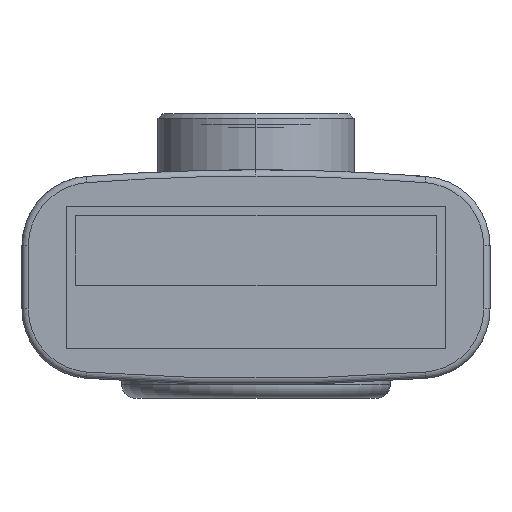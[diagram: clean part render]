
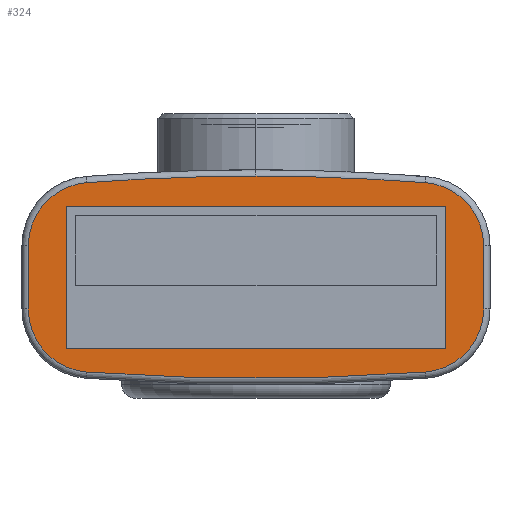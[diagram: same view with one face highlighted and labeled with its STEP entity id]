
A CAD part, front view. The second image highlights one B-rep face of the part: STEP entity #324.
In plain terms, the highlighted planar face has unit normal (0, -1, 0).
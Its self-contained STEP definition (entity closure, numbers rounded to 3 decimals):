
#100 = LINE ( 'NONE', #1617, #2798 ) ;
#133 = CARTESIAN_POINT ( 'NONE',  ( 54.8, -186.8, -10.175 ) ) ;
#142 = CARTESIAN_POINT ( 'NONE',  ( 52.8, -186.8, -12.175 ) ) ;
#231 = AXIS2_PLACEMENT_3D ( 'NONE', #3748, #353, #1868 ) ;
#239 = DIRECTION ( 'NONE',  ( 0., 1., 0. ) ) ;
#260 = CIRCLE ( 'NONE', #338, 69.8 ) ;
#324 = ADVANCED_FACE ( 'NONE', ( #4013, #614 ), #2124, .F. ) ;
#338 = AXIS2_PLACEMENT_3D ( 'NONE', #1811, #3325, #4828 ) ;
#353 = DIRECTION ( 'NONE',  ( 0., 1., 0. ) ) ;
#392 = DIRECTION ( 'NONE',  ( -0.075, 0., -0.997 ) ) ;
#433 = EDGE_CURVE ( 'NONE', #1878, #1006, #3667, .T. ) ;
#448 = CARTESIAN_POINT ( 'NONE',  ( 54., -186.8, -13.425 ) ) ;
#493 = EDGE_CURVE ( 'NONE', #609, #1517, #1768, .T. ) ;
#539 = EDGE_CURVE ( 'NONE', #4317, #609, #260, .T. ) ;
#552 = VERTEX_POINT ( 'NONE', #4093 ) ;
#590 = CARTESIAN_POINT ( 'NONE',  ( 65.2, -186.8, -12.175 ) ) ;
#595 = VERTEX_POINT ( 'NONE', #2628 ) ;
#609 = VERTEX_POINT ( 'NONE', #3400 ) ;
#614 = FACE_BOUND ( 'NONE', #2834, .T. ) ;
#627 = CARTESIAN_POINT ( 'NONE',  ( 52.8, -186.8, -10.176 ) ) ;
#640 = CIRCLE ( 'NONE', #231, 69.8 ) ;
#694 = ORIENTED_EDGE ( 'NONE', *, *, #539, .F. ) ;
#700 = CARTESIAN_POINT ( 'NONE',  ( 65.353, -186.8, -8.181 ) ) ;
#705 = VERTEX_POINT ( 'NONE', #2711 ) ;
#777 = LINE ( 'NONE', #2286, #2953 ) ;
#838 = ORIENTED_EDGE ( 'NONE', *, *, #433, .F. ) ;
#866 = AXIS2_PLACEMENT_3D ( 'NONE', #3635, #239, #1753 ) ;
#899 = DIRECTION ( 'NONE',  ( 0., 0., 1. ) ) ;
#978 = ORIENTED_EDGE ( 'NONE', *, *, #2802, .F. ) ;
#1006 = VERTEX_POINT ( 'NONE', #2347 ) ;
#1067 = AXIS2_PLACEMENT_3D ( 'NONE', #4663, #1274, #2794 ) ;
#1149 = CIRCLE ( 'NONE', #1067, 2. ) ;
#1180 = VERTEX_POINT ( 'NONE', #700 ) ;
#1221 = CARTESIAN_POINT ( 'NONE',  ( 67.2, -186.8, -10.175 ) ) ;
#1274 = DIRECTION ( 'NONE',  ( 0., 1., 0. ) ) ;
#1292 = VECTOR ( 'NONE', #899, 1000. ) ;
#1330 = VERTEX_POINT ( 'NONE', #1221 ) ;
#1357 = EDGE_CURVE ( 'NONE', #4426, #552, #100, .T. ) ;
#1362 = CIRCLE ( 'NONE', #4138, 2. ) ;
#1415 = EDGE_CURVE ( 'NONE', #552, #2485, #2709, .T. ) ;
#1420 = CARTESIAN_POINT ( 'NONE',  ( 54., -186.8, -8.925 ) ) ;
#1517 = VERTEX_POINT ( 'NONE', #142 ) ;
#1617 = CARTESIAN_POINT ( 'NONE',  ( 54., -186.8, -8.925 ) ) ;
#1621 = EDGE_CURVE ( 'NONE', #595, #4317, #3033, .T. ) ;
#1646 = DIRECTION ( 'NONE',  ( 0., 1., 0. ) ) ;
#1753 = DIRECTION ( 'NONE',  ( 1., 0., 0. ) ) ;
#1768 = CIRCLE ( 'NONE', #1845, 2. ) ;
#1771 = VECTOR ( 'NONE', #2135, 1000. ) ;
#1811 = CARTESIAN_POINT ( 'NONE',  ( 60., -186.8, 55.425 ) ) ;
#1841 = VECTOR ( 'NONE', #1961, 1000. ) ;
#1845 = AXIS2_PLACEMENT_3D ( 'NONE', #2282, #3788, #392 ) ;
#1860 = CARTESIAN_POINT ( 'NONE',  ( 60., -186.8, -77.775 ) ) ;
#1868 = DIRECTION ( 'NONE',  ( -0.077, 0., 0.997 ) ) ;
#1878 = VERTEX_POINT ( 'NONE', #4622 ) ;
#1890 = LINE ( 'NONE', #3404, #4301 ) ;
#1961 = DIRECTION ( 'NONE',  ( 1., 0., 0. ) ) ;
#2099 = DIRECTION ( 'NONE',  ( 0., 1., 0. ) ) ;
#2110 = ORIENTED_EDGE ( 'NONE', *, *, #4649, .F. ) ;
#2124 = PLANE ( 'NONE',  #866 ) ;
#2135 = DIRECTION ( 'NONE',  ( 0., 0., -1. ) ) ;
#2282 = CARTESIAN_POINT ( 'NONE',  ( 54.8, -186.8, -12.175 ) ) ;
#2286 = CARTESIAN_POINT ( 'NONE',  ( 67.2, -186.8, -12.174 ) ) ;
#2340 = EDGE_CURVE ( 'NONE', #1180, #1330, #1149, .T. ) ;
#2347 = CARTESIAN_POINT ( 'NONE',  ( 60., -186.8, -7.975 ) ) ;
#2471 = CARTESIAN_POINT ( 'NONE',  ( 65.353, -186.8, -14.169 ) ) ;
#2485 = VERTEX_POINT ( 'NONE', #2894 ) ;
#2497 = EDGE_CURVE ( 'NONE', #705, #1517, #4025, .T. ) ;
#2503 = EDGE_LOOP ( 'NONE', ( #4100, #2891, #838, #2110, #3799, #3072, #694, #4842, #2943 ) ) ;
#2612 = VERTEX_POINT ( 'NONE', #2641 ) ;
#2628 = CARTESIAN_POINT ( 'NONE',  ( 67.2, -186.8, -12.175 ) ) ;
#2641 = CARTESIAN_POINT ( 'NONE',  ( 66., -186.8, -8.925 ) ) ;
#2709 = LINE ( 'NONE', #448, #1841 ) ;
#2711 = CARTESIAN_POINT ( 'NONE',  ( 52.8, -186.8, -10.175 ) ) ;
#2788 = LINE ( 'NONE', #4292, #1292 ) ;
#2794 = DIRECTION ( 'NONE',  ( 0.075, 0., 0.997 ) ) ;
#2798 = VECTOR ( 'NONE', #3138, 1000. ) ;
#2802 = EDGE_CURVE ( 'NONE', #2485, #2612, #2788, .T. ) ;
#2834 = EDGE_LOOP ( 'NONE', ( #978, #4200, #3688, #4092 ) ) ;
#2891 = ORIENTED_EDGE ( 'NONE', *, *, #3414, .F. ) ;
#2894 = CARTESIAN_POINT ( 'NONE',  ( 66., -186.8, -13.425 ) ) ;
#2943 = ORIENTED_EDGE ( 'NONE', *, *, #4887, .T. ) ;
#2953 = VECTOR ( 'NONE', #3792, 1000. ) ;
#3033 = CIRCLE ( 'NONE', #3193, 2. ) ;
#3066 = EDGE_CURVE ( 'NONE', #2612, #4426, #1890, .T. ) ;
#3072 = ORIENTED_EDGE ( 'NONE', *, *, #493, .F. ) ;
#3138 = DIRECTION ( 'NONE',  ( 0., 0., -1. ) ) ;
#3164 = DIRECTION ( 'NONE',  ( -1., 0., -0.002 ) ) ;
#3193 = AXIS2_PLACEMENT_3D ( 'NONE', #590, #2099, #3611 ) ;
#3325 = DIRECTION ( 'NONE',  ( 0., 1., 0. ) ) ;
#3373 = DIRECTION ( 'NONE',  ( 0., 1., 0. ) ) ;
#3400 = CARTESIAN_POINT ( 'NONE',  ( 54.647, -186.8, -14.169 ) ) ;
#3404 = CARTESIAN_POINT ( 'NONE',  ( 66., -186.8, -8.925 ) ) ;
#3414 = EDGE_CURVE ( 'NONE', #1006, #1180, #640, .T. ) ;
#3586 = AXIS2_PLACEMENT_3D ( 'NONE', #1860, #3373, #4873 ) ;
#3611 = DIRECTION ( 'NONE',  ( 1., 0., 0.002 ) ) ;
#3635 = CARTESIAN_POINT ( 'NONE',  ( 60., -186.8, -11.175 ) ) ;
#3667 = CIRCLE ( 'NONE', #3586, 69.8 ) ;
#3688 = ORIENTED_EDGE ( 'NONE', *, *, #1357, .F. ) ;
#3748 = CARTESIAN_POINT ( 'NONE',  ( 60., -186.8, -77.775 ) ) ;
#3788 = DIRECTION ( 'NONE',  ( 0., 1., 0. ) ) ;
#3792 = DIRECTION ( 'NONE',  ( 0., 0., 1. ) ) ;
#3799 = ORIENTED_EDGE ( 'NONE', *, *, #2497, .T. ) ;
#4013 = FACE_OUTER_BOUND ( 'NONE', #2503, .T. ) ;
#4025 = LINE ( 'NONE', #627, #1771 ) ;
#4092 = ORIENTED_EDGE ( 'NONE', *, *, #3066, .F. ) ;
#4093 = CARTESIAN_POINT ( 'NONE',  ( 54., -186.8, -13.425 ) ) ;
#4100 = ORIENTED_EDGE ( 'NONE', *, *, #2340, .F. ) ;
#4138 = AXIS2_PLACEMENT_3D ( 'NONE', #133, #1646, #3164 ) ;
#4200 = ORIENTED_EDGE ( 'NONE', *, *, #1415, .F. ) ;
#4292 = CARTESIAN_POINT ( 'NONE',  ( 66., -186.8, -13.425 ) ) ;
#4301 = VECTOR ( 'NONE', #4904, 1000. ) ;
#4317 = VERTEX_POINT ( 'NONE', #2471 ) ;
#4426 = VERTEX_POINT ( 'NONE', #1420 ) ;
#4622 = CARTESIAN_POINT ( 'NONE',  ( 54.647, -186.8, -8.181 ) ) ;
#4649 = EDGE_CURVE ( 'NONE', #705, #1878, #1362, .T. ) ;
#4663 = CARTESIAN_POINT ( 'NONE',  ( 65.2, -186.8, -10.175 ) ) ;
#4828 = DIRECTION ( 'NONE',  ( 0.077, 0., -0.997 ) ) ;
#4842 = ORIENTED_EDGE ( 'NONE', *, *, #1621, .F. ) ;
#4873 = DIRECTION ( 'NONE',  ( -0.077, 0., 0.997 ) ) ;
#4887 = EDGE_CURVE ( 'NONE', #595, #1330, #777, .T. ) ;
#4904 = DIRECTION ( 'NONE',  ( -1., 0., 0. ) ) ;
